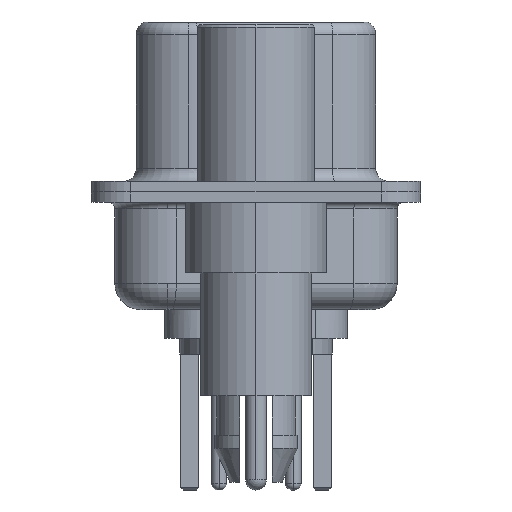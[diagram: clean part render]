
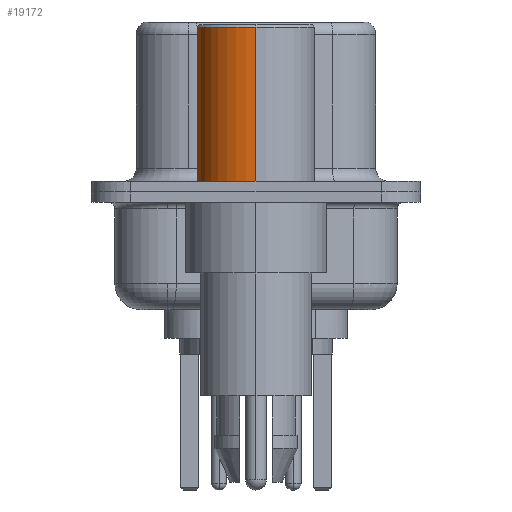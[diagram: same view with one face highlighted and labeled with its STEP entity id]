
A CAD part, left-side view. The second image highlights one B-rep face of the part: STEP entity #19172.
In plain terms, the highlighted cylindrical face has radius 2.25 mm (diameter 4.5 mm), a partial arc.
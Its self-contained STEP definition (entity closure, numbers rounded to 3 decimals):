
#214 = AXIS2_PLACEMENT_3D ( 'NONE', #8974, #13161, #6523 ) ;
#782 = ORIENTED_EDGE ( 'NONE', *, *, #2380, .F. ) ;
#1469 = CARTESIAN_POINT ( 'NONE',  ( 2.25, 0., 6.3 ) ) ;
#1923 = LINE ( 'NONE', #19890, #17999 ) ;
#1956 = CARTESIAN_POINT ( 'NONE',  ( 2.25, 0., 0.4 ) ) ;
#2168 = EDGE_CURVE ( 'NONE', #8853, #5663, #19355, .T. ) ;
#2343 = EDGE_CURVE ( 'NONE', #13087, #4602, #10816, .T. ) ;
#2375 = EDGE_CURVE ( 'NONE', #4602, #5663, #18465, .T. ) ;
#2380 = EDGE_CURVE ( 'NONE', #13087, #8853, #1923, .T. ) ;
#2414 = ORIENTED_EDGE ( 'NONE', *, *, #2375, .T. ) ;
#3512 = CARTESIAN_POINT ( 'NONE',  ( 0., 0., 0.581 ) ) ;
#4584 = EDGE_LOOP ( 'NONE', ( #8044, #2414, #11578, #782 ) ) ;
#4602 = VERTEX_POINT ( 'NONE', #13502 ) ;
#5161 = DIRECTION ( 'NONE',  ( 0., 0., 1. ) ) ;
#5195 = FACE_OUTER_BOUND ( 'NONE', #4584, .T. ) ;
#5663 = VERTEX_POINT ( 'NONE', #12311 ) ;
#6523 = DIRECTION ( 'NONE',  ( 1., 0., 0. ) ) ;
#7589 = AXIS2_PLACEMENT_3D ( 'NONE', #3512, #5161, #14393 ) ;
#8044 = ORIENTED_EDGE ( 'NONE', *, *, #2343, .T. ) ;
#8841 = CARTESIAN_POINT ( 'NONE',  ( 0., 0., 0.4 ) ) ;
#8853 = VERTEX_POINT ( 'NONE', #1469 ) ;
#8861 = CYLINDRICAL_SURFACE ( 'NONE', #7589, 2.25 ) ;
#8974 = CARTESIAN_POINT ( 'NONE',  ( 0., 0., 6.3 ) ) ;
#9521 = DIRECTION ( 'NONE',  ( 1., 0., 0. ) ) ;
#9904 = DIRECTION ( 'NONE',  ( 0., 0., 1. ) ) ;
#10468 = CARTESIAN_POINT ( 'NONE',  ( -2.25, 0., 0.581 ) ) ;
#10816 = CIRCLE ( 'NONE', #12162, 2.25 ) ;
#11578 = ORIENTED_EDGE ( 'NONE', *, *, #2168, .F. ) ;
#12162 = AXIS2_PLACEMENT_3D ( 'NONE', #8841, #16024, #9521 ) ;
#12311 = CARTESIAN_POINT ( 'NONE',  ( -2.25, 0., 6.3 ) ) ;
#13087 = VERTEX_POINT ( 'NONE', #1956 ) ;
#13161 = DIRECTION ( 'NONE',  ( 0., 0., 1. ) ) ;
#13502 = CARTESIAN_POINT ( 'NONE',  ( -2.25, 0., 0.4 ) ) ;
#13926 = VECTOR ( 'NONE', #9904, 1000. ) ;
#14393 = DIRECTION ( 'NONE',  ( 1., 0., 0. ) ) ;
#16024 = DIRECTION ( 'NONE',  ( 0., 0., 1. ) ) ;
#17999 = VECTOR ( 'NONE', #18497, 1000. ) ;
#18465 = LINE ( 'NONE', #10468, #13926 ) ;
#18497 = DIRECTION ( 'NONE',  ( 0., 0., 1. ) ) ;
#19172 = ADVANCED_FACE ( 'NONE', ( #5195 ), #8861, .T. ) ;
#19355 = CIRCLE ( 'NONE', #214, 2.25 ) ;
#19890 = CARTESIAN_POINT ( 'NONE',  ( 2.25, 0., 0.581 ) ) ;
